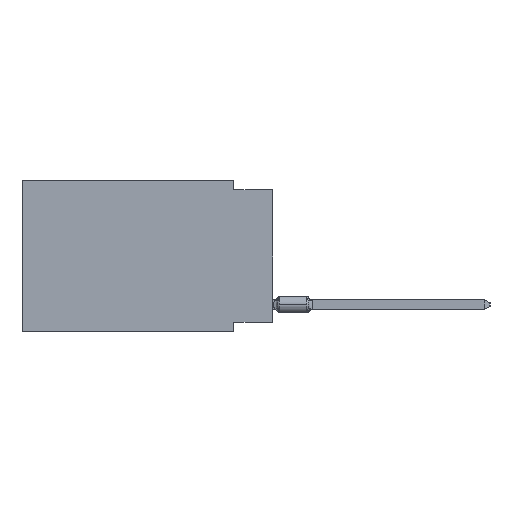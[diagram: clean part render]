
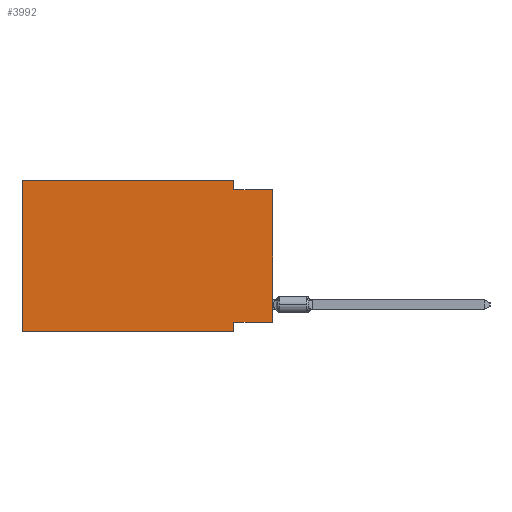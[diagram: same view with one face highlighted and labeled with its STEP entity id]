
A CAD part, left-side view. The second image highlights one B-rep face of the part: STEP entity #3992.
In plain terms, the highlighted planar face has unit normal (-1, 0, 0).
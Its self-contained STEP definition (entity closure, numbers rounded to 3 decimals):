
#52 = CARTESIAN_POINT ( 'NONE',  ( 0., 2.54, -9.906 ) ) ;
#945 = FACE_OUTER_BOUND ( 'NONE', #71907, .T. ) ;
#1377 = ORIENTED_EDGE ( 'NONE', *, *, #39141, .T. ) ;
#3131 = DIRECTION ( 'NONE',  ( 0., -1., 0. ) ) ;
#3992 = ADVANCED_FACE ( 'NONE', ( #945 ), #34169, .F. ) ;
#4357 = DIRECTION ( 'NONE',  ( 0., -1., 0. ) ) ;
#4428 = ORIENTED_EDGE ( 'NONE', *, *, #55618, .T. ) ;
#4680 = LINE ( 'NONE', #17210, #45835 ) ;
#5006 = DIRECTION ( 'NONE',  ( 0., -1., 0. ) ) ;
#5614 = VERTEX_POINT ( 'NONE', #12977 ) ;
#6078 = EDGE_CURVE ( 'NONE', #17018, #66131, #39174, .T. ) ;
#7854 = DIRECTION ( 'NONE',  ( 0., 0., -1. ) ) ;
#8838 = DIRECTION ( 'NONE',  ( 0., 1., 0. ) ) ;
#9261 = LINE ( 'NONE', #75297, #52371 ) ;
#9609 = LINE ( 'NONE', #62249, #63763 ) ;
#10231 = CARTESIAN_POINT ( 'NONE',  ( 0., 0., -9.271 ) ) ;
#10242 = EDGE_CURVE ( 'NONE', #66131, #5614, #63483, .T. ) ;
#10750 = DIRECTION ( 'NONE',  ( 0., 0., 1. ) ) ;
#11758 = CARTESIAN_POINT ( 'NONE',  ( 0., 2.54, -0.635 ) ) ;
#12432 = ORIENTED_EDGE ( 'NONE', *, *, #60466, .F. ) ;
#12977 = CARTESIAN_POINT ( 'NONE',  ( 0., 0., -0.635 ) ) ;
#13905 = DIRECTION ( 'NONE',  ( 1., 0., 0. ) ) ;
#14755 = CARTESIAN_POINT ( 'NONE',  ( 0., 16.383, 0. ) ) ;
#15399 = DIRECTION ( 'NONE',  ( 0., 0., -1. ) ) ;
#16898 = ORIENTED_EDGE ( 'NONE', *, *, #10242, .F. ) ;
#17018 = VERTEX_POINT ( 'NONE', #67828 ) ;
#17210 = CARTESIAN_POINT ( 'NONE',  ( 0., 0., 0. ) ) ;
#18816 = CARTESIAN_POINT ( 'NONE',  ( 0., 16.383, -9.906 ) ) ;
#23760 = ORIENTED_EDGE ( 'NONE', *, *, #52345, .F. ) ;
#24094 = DIRECTION ( 'NONE',  ( 0., 0., 1. ) ) ;
#29753 = LINE ( 'NONE', #50023, #84744 ) ;
#30452 = CARTESIAN_POINT ( 'NONE',  ( 0., 2.54, -9.271 ) ) ;
#32522 = VECTOR ( 'NONE', #73818, 1000. ) ;
#34169 = PLANE ( 'NONE',  #60977 ) ;
#34403 = CARTESIAN_POINT ( 'NONE',  ( 0., 2.54, 0. ) ) ;
#35346 = VERTEX_POINT ( 'NONE', #10231 ) ;
#39141 = EDGE_CURVE ( 'NONE', #73081, #78785, #64144, .T. ) ;
#39174 = LINE ( 'NONE', #34403, #51547 ) ;
#39324 = EDGE_CURVE ( 'NONE', #35346, #68464, #9261, .T. ) ;
#40857 = ORIENTED_EDGE ( 'NONE', *, *, #6078, .F. ) ;
#41395 = CARTESIAN_POINT ( 'NONE',  ( 0., 16.383, 0. ) ) ;
#42330 = CARTESIAN_POINT ( 'NONE',  ( 0., 0., -0.635 ) ) ;
#43012 = CARTESIAN_POINT ( 'NONE',  ( 0., 16.383, -9.906 ) ) ;
#43636 = ORIENTED_EDGE ( 'NONE', *, *, #69167, .F. ) ;
#45835 = VECTOR ( 'NONE', #24094, 1000. ) ;
#46207 = ORIENTED_EDGE ( 'NONE', *, *, #39324, .F. ) ;
#47891 = LINE ( 'NONE', #72963, #32522 ) ;
#50023 = CARTESIAN_POINT ( 'NONE',  ( 0., 16.383, 0. ) ) ;
#51547 = VECTOR ( 'NONE', #15399, 1000. ) ;
#52345 = EDGE_CURVE ( 'NONE', #57654, #17018, #9609, .T. ) ;
#52371 = VECTOR ( 'NONE', #8838, 1000. ) ;
#55618 = EDGE_CURVE ( 'NONE', #35346, #5614, #4680, .T. ) ;
#57654 = VERTEX_POINT ( 'NONE', #41395 ) ;
#60466 = EDGE_CURVE ( 'NONE', #68464, #78785, #47891, .T. ) ;
#60977 = AXIS2_PLACEMENT_3D ( 'NONE', #14755, #13905, #7854 ) ;
#62039 = VECTOR ( 'NONE', #5006, 1000. ) ;
#62249 = CARTESIAN_POINT ( 'NONE',  ( 0., 16.383, 0. ) ) ;
#63483 = LINE ( 'NONE', #42330, #73860 ) ;
#63763 = VECTOR ( 'NONE', #3131, 1000. ) ;
#64144 = LINE ( 'NONE', #18816, #62039 ) ;
#66131 = VERTEX_POINT ( 'NONE', #11758 ) ;
#67828 = CARTESIAN_POINT ( 'NONE',  ( 0., 2.54, 0. ) ) ;
#68464 = VERTEX_POINT ( 'NONE', #30452 ) ;
#69167 = EDGE_CURVE ( 'NONE', #73081, #57654, #29753, .T. ) ;
#71907 = EDGE_LOOP ( 'NONE', ( #4428, #16898, #40857, #23760, #43636, #1377, #12432, #46207 ) ) ;
#72963 = CARTESIAN_POINT ( 'NONE',  ( 0., 2.54, -9.906 ) ) ;
#73081 = VERTEX_POINT ( 'NONE', #43012 ) ;
#73818 = DIRECTION ( 'NONE',  ( 0., 0., -1. ) ) ;
#73860 = VECTOR ( 'NONE', #4357, 1000. ) ;
#75297 = CARTESIAN_POINT ( 'NONE',  ( 0., 0., -9.271 ) ) ;
#78785 = VERTEX_POINT ( 'NONE', #52 ) ;
#84744 = VECTOR ( 'NONE', #10750, 1000. ) ;
